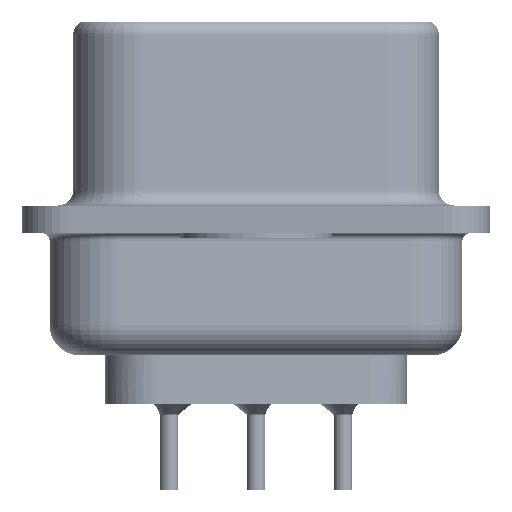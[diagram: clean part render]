
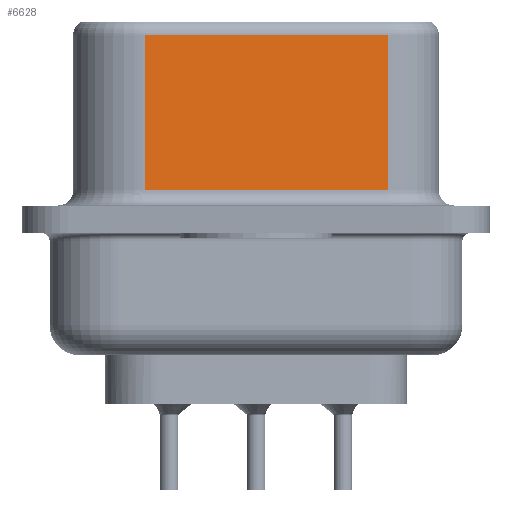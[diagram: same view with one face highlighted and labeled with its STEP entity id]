
A CAD part, left-side view. The second image highlights one B-rep face of the part: STEP entity #6628.
In plain terms, the highlighted planar face has unit normal (-0.985, -0.174, 0).
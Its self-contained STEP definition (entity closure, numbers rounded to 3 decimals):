
#17 = VERTEX_POINT ( 'NONE', #23819 ) ;
#553 = PLANE ( 'NONE',  #17405 ) ;
#1612 = VERTEX_POINT ( 'NONE', #8942 ) ;
#2390 = VECTOR ( 'NONE', #29639, 1000. ) ;
#2401 = VECTOR ( 'NONE', #18713, 1000. ) ;
#2802 = CARTESIAN_POINT ( 'NONE',  ( 5.132, -4.322, 6.02 ) ) ;
#5058 = VERTEX_POINT ( 'NONE', #32036 ) ;
#5752 = CARTESIAN_POINT ( 'NONE',  ( 5.132, -4.322, 6.52 ) ) ;
#6227 = DIRECTION ( 'NONE',  ( 0., 0., -1. ) ) ;
#6628 = ADVANCED_FACE ( 'NONE', ( #33480 ), #553, .F. ) ;
#8376 = ORIENTED_EDGE ( 'NONE', *, *, #22074, .F. ) ;
#8433 = DIRECTION ( 'NONE',  ( -0.174, 0.985, 0. ) ) ;
#8942 = CARTESIAN_POINT ( 'NONE',  ( 3.73, 3.628, 0.95 ) ) ;
#9064 = LINE ( 'NONE', #24472, #14399 ) ;
#9388 = LINE ( 'NONE', #28833, #2401 ) ;
#9753 = ORIENTED_EDGE ( 'NONE', *, *, #25119, .T. ) ;
#9890 = EDGE_CURVE ( 'NONE', #1612, #5058, #9388, .T. ) ;
#14399 = VECTOR ( 'NONE', #6227, 1000. ) ;
#17405 = AXIS2_PLACEMENT_3D ( 'NONE', #5752, #23995, #8433 ) ;
#18713 = DIRECTION ( 'NONE',  ( 0.174, -0.985, 0. ) ) ;
#20421 = EDGE_CURVE ( 'NONE', #22049, #1612, #9064, .T. ) ;
#20470 = LINE ( 'NONE', #2802, #27305 ) ;
#20759 = LINE ( 'NONE', #27068, #2390 ) ;
#22049 = VERTEX_POINT ( 'NONE', #29520 ) ;
#22074 = EDGE_CURVE ( 'NONE', #17, #5058, #20759, .T. ) ;
#23665 = DIRECTION ( 'NONE',  ( -0.174, 0.985, 0. ) ) ;
#23819 = CARTESIAN_POINT ( 'NONE',  ( 5.132, -4.322, 6.02 ) ) ;
#23995 = DIRECTION ( 'NONE',  ( 0.985, 0.174, 0. ) ) ;
#24422 = ORIENTED_EDGE ( 'NONE', *, *, #9890, .T. ) ;
#24472 = CARTESIAN_POINT ( 'NONE',  ( 3.73, 3.628, 6.52 ) ) ;
#25119 = EDGE_CURVE ( 'NONE', #17, #22049, #20470, .T. ) ;
#26083 = EDGE_LOOP ( 'NONE', ( #8376, #9753, #33213, #24422 ) ) ;
#27068 = CARTESIAN_POINT ( 'NONE',  ( 5.132, -4.322, 6.52 ) ) ;
#27305 = VECTOR ( 'NONE', #23665, 1000. ) ;
#28833 = CARTESIAN_POINT ( 'NONE',  ( 5.132, -4.322, 0.95 ) ) ;
#29520 = CARTESIAN_POINT ( 'NONE',  ( 3.73, 3.628, 6.02 ) ) ;
#29639 = DIRECTION ( 'NONE',  ( 0., 0., -1. ) ) ;
#32036 = CARTESIAN_POINT ( 'NONE',  ( 5.132, -4.322, 0.95 ) ) ;
#33213 = ORIENTED_EDGE ( 'NONE', *, *, #20421, .T. ) ;
#33480 = FACE_OUTER_BOUND ( 'NONE', #26083, .T. ) ;
